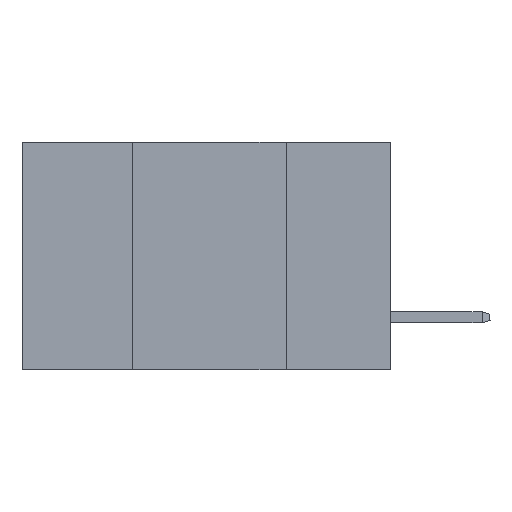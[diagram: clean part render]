
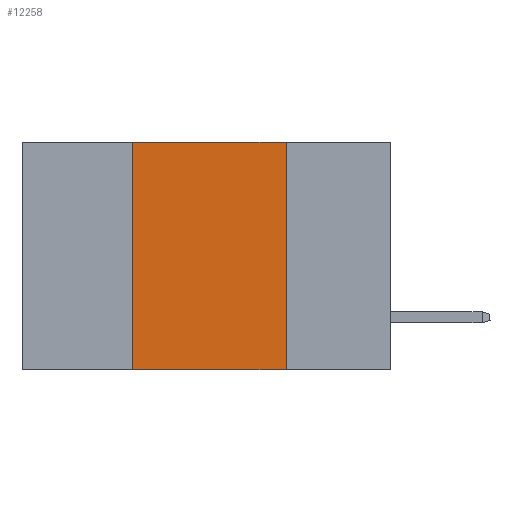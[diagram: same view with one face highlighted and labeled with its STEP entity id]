
A CAD part, left-side view. The second image highlights one B-rep face of the part: STEP entity #12258.
In plain terms, the highlighted planar face has unit normal (-1, 0, 0).
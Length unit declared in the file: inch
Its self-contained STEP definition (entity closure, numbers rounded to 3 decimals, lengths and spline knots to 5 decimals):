
#1331 = CARTESIAN_POINT ( 'NONE',  ( 0., 0.17, 0. ) ) ;
#1418 = DIRECTION ( 'NONE',  ( 0., 0., -1. ) ) ;
#3263 = ORIENTED_EDGE ( 'NONE', *, *, #23140, .F. ) ;
#3868 = CARTESIAN_POINT ( 'NONE',  ( 0., 0.6, 0. ) ) ;
#4069 = DIRECTION ( 'NONE',  ( 1., 0., 0. ) ) ;
#4443 = ORIENTED_EDGE ( 'NONE', *, *, #13018, .F. ) ;
#5537 = CARTESIAN_POINT ( 'NONE',  ( 0., 0.17, 0. ) ) ;
#5746 = CARTESIAN_POINT ( 'NONE',  ( 0., 0.17, -0.37 ) ) ;
#5947 = ORIENTED_EDGE ( 'NONE', *, *, #22067, .T. ) ;
#7885 = VECTOR ( 'NONE', #11590, 39.37008 ) ;
#8009 = VERTEX_POINT ( 'NONE', #19167 ) ;
#9617 = LINE ( 'NONE', #1331, #22202 ) ;
#9794 = DIRECTION ( 'NONE',  ( 0., -1., 0. ) ) ;
#10099 = PLANE ( 'NONE',  #14111 ) ;
#10376 = CARTESIAN_POINT ( 'NONE',  ( 0., 0.6, 0. ) ) ;
#11486 = LINE ( 'NONE', #3868, #14863 ) ;
#11590 = DIRECTION ( 'NONE',  ( 0., -1., 0. ) ) ;
#11674 = CARTESIAN_POINT ( 'NONE',  ( 0., 0.6, -0.37 ) ) ;
#11763 = EDGE_LOOP ( 'NONE', ( #18011, #4443, #3263, #5947 ) ) ;
#12229 = CARTESIAN_POINT ( 'NONE',  ( 0., 0.42, -0.37 ) ) ;
#12258 = ADVANCED_FACE ( 'NONE', ( #14580 ), #10099, .F. ) ;
#13018 = EDGE_CURVE ( 'NONE', #8009, #17306, #11486, .T. ) ;
#14111 = AXIS2_PLACEMENT_3D ( 'NONE', #10376, #4069, #27156 ) ;
#14580 = FACE_OUTER_BOUND ( 'NONE', #11763, .T. ) ;
#14863 = VECTOR ( 'NONE', #9794, 39.37008 ) ;
#16212 = EDGE_CURVE ( 'NONE', #17306, #20944, #9617, .T. ) ;
#17306 = VERTEX_POINT ( 'NONE', #5537 ) ;
#18011 = ORIENTED_EDGE ( 'NONE', *, *, #16212, .F. ) ;
#19167 = CARTESIAN_POINT ( 'NONE',  ( 0., 0.42, 0. ) ) ;
#20142 = DIRECTION ( 'NONE',  ( 0., 0., 1. ) ) ;
#20765 = LINE ( 'NONE', #26385, #26776 ) ;
#20944 = VERTEX_POINT ( 'NONE', #5746 ) ;
#22067 = EDGE_CURVE ( 'NONE', #26510, #20944, #25825, .T. ) ;
#22202 = VECTOR ( 'NONE', #1418, 39.37008 ) ;
#23140 = EDGE_CURVE ( 'NONE', #26510, #8009, #20765, .T. ) ;
#25825 = LINE ( 'NONE', #11674, #7885 ) ;
#26385 = CARTESIAN_POINT ( 'NONE',  ( 0., 0.42, 0. ) ) ;
#26510 = VERTEX_POINT ( 'NONE', #12229 ) ;
#26776 = VECTOR ( 'NONE', #20142, 39.37008 ) ;
#27156 = DIRECTION ( 'NONE',  ( 0., 0., -1. ) ) ;
